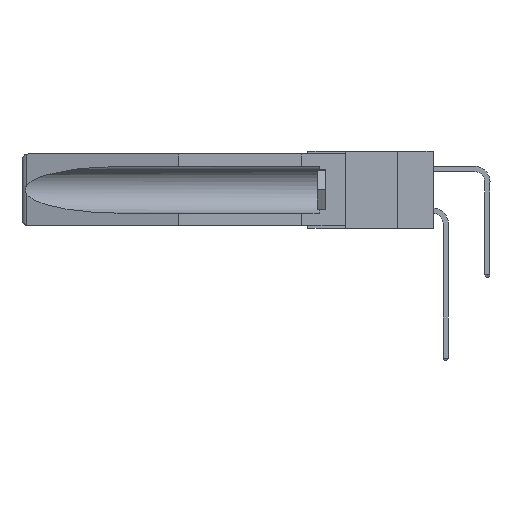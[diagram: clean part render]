
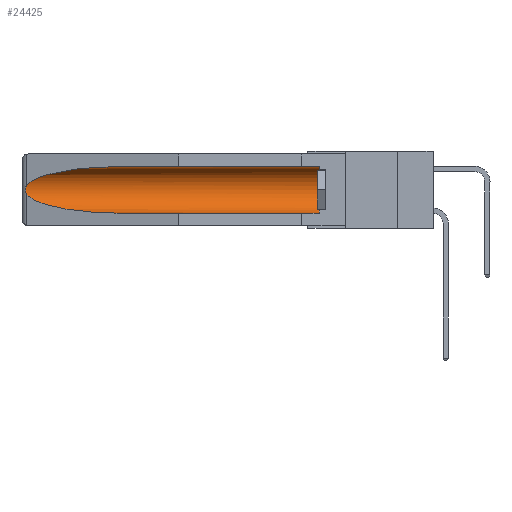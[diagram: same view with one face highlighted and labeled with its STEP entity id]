
A CAD part, left-side view. The second image highlights one B-rep face of the part: STEP entity #24425.
In plain terms, the highlighted cylindrical face has radius 2.857 mm (diameter 5.715 mm), a partial arc.
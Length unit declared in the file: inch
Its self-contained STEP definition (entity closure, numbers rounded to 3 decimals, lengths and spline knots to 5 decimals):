
#73 = VERTEX_POINT ( 'NONE', #25828 ) ;
#86 = CARTESIAN_POINT ( 'NONE',  ( 0.155, 1.07973, -0.284 ) ) ;
#1118 = CARTESIAN_POINT ( 'NONE',  ( 0.2675, 1.53308, -0.16763 ) ) ;
#1555 = CARTESIAN_POINT ( 'NONE',  ( 0.26537, 1.52718, -0.14972 ) ) ;
#2067 = EDGE_CURVE ( 'NONE', #11728, #25368, #12016, .T. ) ;
#2153 = CARTESIAN_POINT ( 'NONE',  ( 0.21114, 1.30732, -0.284 ) ) ;
#2154 = DIRECTION ( 'NONE',  ( 0., 1., 0. ) ) ;
#3491 = CARTESIAN_POINT ( 'NONE',  ( 0.2673, 1.53269, -0.17917 ) ) ;
#4028 = CARTESIAN_POINT ( 'NONE',  ( 0.26537, 1.52718, -0.19328 ) ) ;
#4459 = CYLINDRICAL_SURFACE ( 'NONE', #19411, 0.1125 ) ;
#5694 = CARTESIAN_POINT ( 'NONE',  ( 0.2673, 1.5327, -0.16383 ) ) ;
#7378 = CARTESIAN_POINT ( 'NONE',  ( 0.25451, 1.48313, -0.09465 ) ) ;
#7493 = CARTESIAN_POINT ( 'NONE',  ( 0.26537, 1.52718, -0.14972 ) ) ;
#7540 = ORIENTED_EDGE ( 'NONE', *, *, #8692, .T. ) ;
#7742 = VERTEX_POINT ( 'NONE', #4028 ) ;
#8272 = CARTESIAN_POINT ( 'NONE',  ( 0.26597, 1.5296, -0.19026 ) ) ;
#8692 = EDGE_CURVE ( 'NONE', #11728, #24372, #25395, .T. ) ;
#9009 = ORIENTED_EDGE ( 'NONE', *, *, #17061, .T. ) ;
#9149 = B_SPLINE_CURVE_WITH_KNOTS ( 'NONE', 3,
 ( #17107, #16900, #15268, #5694, #1118, #22121, #3491, #17786, #8272, #19972 ),
 .UNSPECIFIED., .F., .F.,
 ( 4, 2, 2, 2, 4 ),
 ( 0., 0.00029, 0.00058, 0.00087, 0.00117 ),
 .UNSPECIFIED. ) ;
#9156 = EDGE_CURVE ( 'NONE', #7742, #25368, #23275, .T. ) ;
#9528 = ORIENTED_EDGE ( 'NONE', *, *, #9156, .T. ) ;
#9591 = AXIS2_PLACEMENT_3D ( 'NONE', #11607, #20726, #23401 ) ;
#11075 = CARTESIAN_POINT ( 'NONE',  ( 0.155, 0.126, -0.059 ) ) ;
#11607 = CARTESIAN_POINT ( 'NONE',  ( 0.155, 0.126, -0.1715 ) ) ;
#11728 = VERTEX_POINT ( 'NONE', #22513 ) ;
#12016 = LINE ( 'NONE', #22953, #24861 ) ;
#12018 = CARTESIAN_POINT ( 'NONE',  ( 0.155, -0.30754, -0.059 ) ) ;
#12896 = EDGE_CURVE ( 'NONE', #24372, #73, #26500, .T. ) ;
#14003 = VECTOR ( 'NONE', #14307, 39.37008 ) ;
#14307 = DIRECTION ( 'NONE',  ( 0., 1., 0. ) ) ;
#14863 = ORIENTED_EDGE ( 'NONE', *, *, #2067, .F. ) ;
#15268 = CARTESIAN_POINT ( 'NONE',  ( 0.26654, 1.53092, -0.15636 ) ) ;
#15987 = DIRECTION ( 'NONE',  ( 0., 0., 1. ) ) ;
#16517 = CARTESIAN_POINT ( 'NONE',  ( 0.155, 1.07973, -0.059 ) ) ;
#16900 = CARTESIAN_POINT ( 'NONE',  ( 0.26597, 1.52961, -0.15275 ) ) ;
#17061 = EDGE_CURVE ( 'NONE', #25837, #7742, #9149, .T. ) ;
#17107 = CARTESIAN_POINT ( 'NONE',  ( 0.26537, 1.52718, -0.14972 ) ) ;
#17786 = CARTESIAN_POINT ( 'NONE',  ( 0.26655, 1.53094, -0.18657 ) ) ;
#19411 = AXIS2_PLACEMENT_3D ( 'NONE', #30455, #2154, #15987 ) ;
#19972 = CARTESIAN_POINT ( 'NONE',  ( 0.26537, 1.52718, -0.19328 ) ) ;
#20726 = DIRECTION ( 'NONE',  ( 0., -1., 0. ) ) ;
#20893 = CARTESIAN_POINT ( 'NONE',  ( 0.26537, 1.52718, -0.19328 ) ) ;
#21756 = EDGE_LOOP ( 'NONE', ( #30101, #9009, #9528, #14863, #7540, #21969 ) ) ;
#21969 = ORIENTED_EDGE ( 'NONE', *, *, #12896, .T. ) ;
#22121 = CARTESIAN_POINT ( 'NONE',  ( 0.2675, 1.53308, -0.17534 ) ) ;
#22513 = CARTESIAN_POINT ( 'NONE',  ( 0.155, 0.126, -0.284 ) ) ;
#22953 = CARTESIAN_POINT ( 'NONE',  ( 0.155, -0.30754, -0.284 ) ) ;
#23058 = CARTESIAN_POINT ( 'NONE',  ( 0.155, 1.07973, -0.284 ) ) ;
#23275 =( BOUNDED_CURVE ( )  B_SPLINE_CURVE ( 3, ( #20893, #25623, #2153, #86 ),
 .UNSPECIFIED., .F., .F. ) 
 B_SPLINE_CURVE_WITH_KNOTS ( ( 4, 4 ),
 ( 0.1948, 1.5708 ),
 .UNSPECIFIED. ) 
 CURVE ( )  GEOMETRIC_REPRESENTATION_ITEM ( )  RATIONAL_B_SPLINE_CURVE ( ( 1., 0.848, 0.848, 1. ) ) 
 REPRESENTATION_ITEM ( '' )  );
#23401 = DIRECTION ( 'NONE',  ( 0., 0., 1. ) ) ;
#23668 =( BOUNDED_CURVE ( )  B_SPLINE_CURVE ( 3, ( #16517, #28122, #7378, #7493 ),
 .UNSPECIFIED., .F., .T. ) 
 B_SPLINE_CURVE_WITH_KNOTS ( ( 4, 4 ),
 ( 4.71239, 6.08839 ),
 .UNSPECIFIED. ) 
 CURVE ( )  GEOMETRIC_REPRESENTATION_ITEM ( )  RATIONAL_B_SPLINE_CURVE ( ( 1., 0.848, 0.848, 1. ) ) 
 REPRESENTATION_ITEM ( '' )  );
#24372 = VERTEX_POINT ( 'NONE', #11075 ) ;
#24425 = ADVANCED_FACE ( 'NONE', ( #25781 ), #4459, .F. ) ;
#24861 = VECTOR ( 'NONE', #27686, 39.37008 ) ;
#25368 = VERTEX_POINT ( 'NONE', #23058 ) ;
#25395 = CIRCLE ( 'NONE', #9591, 0.1125 ) ;
#25623 = CARTESIAN_POINT ( 'NONE',  ( 0.25451, 1.48313, -0.24835 ) ) ;
#25781 = FACE_OUTER_BOUND ( 'NONE', #21756, .T. ) ;
#25828 = CARTESIAN_POINT ( 'NONE',  ( 0.155, 1.07973, -0.059 ) ) ;
#25837 = VERTEX_POINT ( 'NONE', #1555 ) ;
#26500 = LINE ( 'NONE', #12018, #14003 ) ;
#27686 = DIRECTION ( 'NONE',  ( 0., 1., 0. ) ) ;
#28122 = CARTESIAN_POINT ( 'NONE',  ( 0.21114, 1.30732, -0.059 ) ) ;
#29211 = EDGE_CURVE ( 'NONE', #73, #25837, #23668, .T. ) ;
#30101 = ORIENTED_EDGE ( 'NONE', *, *, #29211, .T. ) ;
#30455 = CARTESIAN_POINT ( 'NONE',  ( 0.155, -0.30754, -0.1715 ) ) ;
